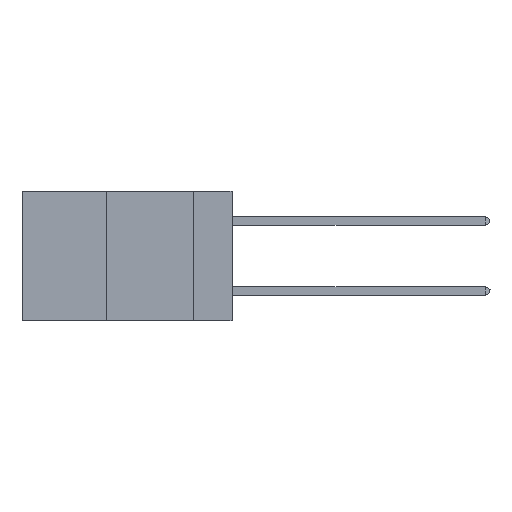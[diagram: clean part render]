
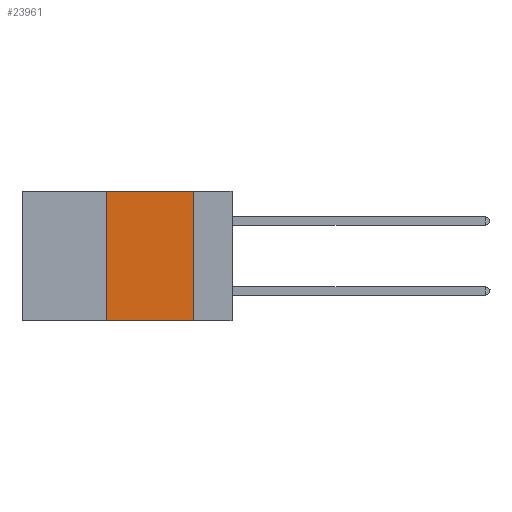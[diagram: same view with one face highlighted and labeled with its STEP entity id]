
A CAD part, left-side view. The second image highlights one B-rep face of the part: STEP entity #23961.
In plain terms, the highlighted planar face has unit normal (-1, 0, 0).
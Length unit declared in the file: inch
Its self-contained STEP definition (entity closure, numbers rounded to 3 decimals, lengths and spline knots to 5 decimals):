
#102 = EDGE_CURVE ( 'NONE', #22692, #16709, #6818, .T. ) ;
#1086 = EDGE_CURVE ( 'NONE', #36169, #13522, #25119, .T. ) ;
#1420 = CARTESIAN_POINT ( 'NONE',  ( 0., 0.11, 0. ) ) ;
#2926 = VECTOR ( 'NONE', #36287, 39.37008 ) ;
#2967 = DIRECTION ( 'NONE',  ( 0., 0., 1. ) ) ;
#3870 = CARTESIAN_POINT ( 'NONE',  ( 0., 0.6, 0. ) ) ;
#3952 = LINE ( 'NONE', #36929, #7793 ) ;
#5243 = EDGE_CURVE ( 'NONE', #22692, #36169, #3952, .T. ) ;
#6043 = AXIS2_PLACEMENT_3D ( 'NONE', #37425, #9829, #12808 ) ;
#6818 = LINE ( 'NONE', #19948, #2926 ) ;
#7350 = ORIENTED_EDGE ( 'NONE', *, *, #14420, .F. ) ;
#7581 = CARTESIAN_POINT ( 'NONE',  ( 0., 0.36, 0. ) ) ;
#7793 = VECTOR ( 'NONE', #2967, 39.37008 ) ;
#8439 = EDGE_LOOP ( 'NONE', ( #7350, #21008, #31053, #11709 ) ) ;
#9829 = DIRECTION ( 'NONE',  ( 1., 0., 0. ) ) ;
#10357 = DIRECTION ( 'NONE',  ( 0., -1., 0. ) ) ;
#11709 = ORIENTED_EDGE ( 'NONE', *, *, #102, .T. ) ;
#12808 = DIRECTION ( 'NONE',  ( 0., 0., -1. ) ) ;
#13066 = LINE ( 'NONE', #1420, #34332 ) ;
#13522 = VERTEX_POINT ( 'NONE', #15756 ) ;
#14420 = EDGE_CURVE ( 'NONE', #13522, #16709, #13066, .T. ) ;
#15756 = CARTESIAN_POINT ( 'NONE',  ( 0., 0.11, 0. ) ) ;
#15931 = PLANE ( 'NONE',  #6043 ) ;
#16709 = VERTEX_POINT ( 'NONE', #28507 ) ;
#18063 = FACE_OUTER_BOUND ( 'NONE', #8439, .T. ) ;
#19948 = CARTESIAN_POINT ( 'NONE',  ( 0., 0.6, -0.37 ) ) ;
#21008 = ORIENTED_EDGE ( 'NONE', *, *, #1086, .F. ) ;
#22692 = VERTEX_POINT ( 'NONE', #34411 ) ;
#23961 = ADVANCED_FACE ( 'NONE', ( #18063 ), #15931, .F. ) ;
#25119 = LINE ( 'NONE', #3870, #26563 ) ;
#26173 = DIRECTION ( 'NONE',  ( 0., 0., -1. ) ) ;
#26563 = VECTOR ( 'NONE', #10357, 39.37008 ) ;
#28507 = CARTESIAN_POINT ( 'NONE',  ( 0., 0.11, -0.37 ) ) ;
#31053 = ORIENTED_EDGE ( 'NONE', *, *, #5243, .F. ) ;
#34332 = VECTOR ( 'NONE', #26173, 39.37008 ) ;
#34411 = CARTESIAN_POINT ( 'NONE',  ( 0., 0.36, -0.37 ) ) ;
#36169 = VERTEX_POINT ( 'NONE', #7581 ) ;
#36287 = DIRECTION ( 'NONE',  ( 0., -1., 0. ) ) ;
#36929 = CARTESIAN_POINT ( 'NONE',  ( 0., 0.36, 0. ) ) ;
#37425 = CARTESIAN_POINT ( 'NONE',  ( 0., 0.6, 0. ) ) ;
